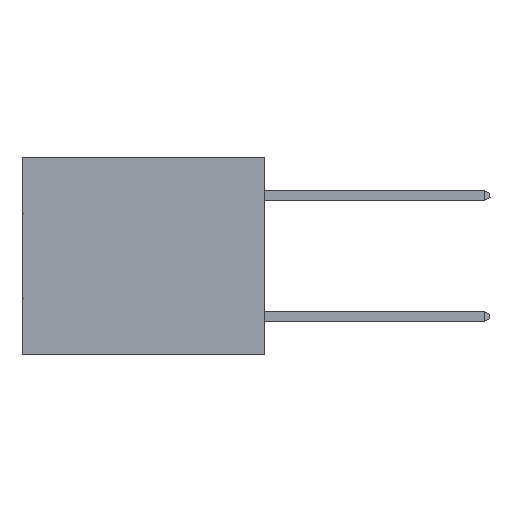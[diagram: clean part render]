
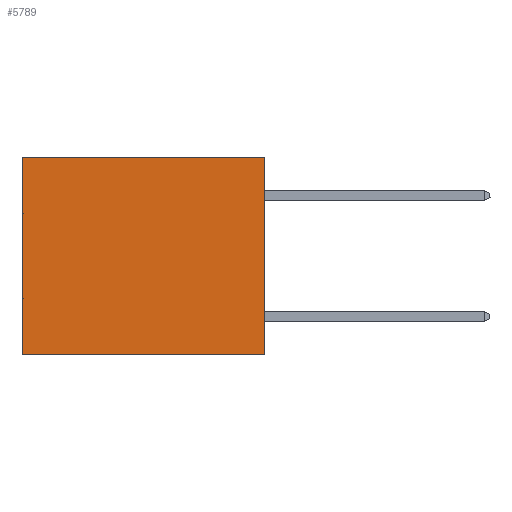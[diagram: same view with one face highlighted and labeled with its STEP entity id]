
A CAD part, left-side view. The second image highlights one B-rep face of the part: STEP entity #5789.
In plain terms, the highlighted planar face has unit normal (-1, 0, 0).
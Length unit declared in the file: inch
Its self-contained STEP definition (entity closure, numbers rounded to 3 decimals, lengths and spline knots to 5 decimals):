
#2473 = EDGE_CURVE ( 'NONE', #23734, #28586, #5473, .T. ) ;
#2545 = VERTEX_POINT ( 'NONE', #25136 ) ;
#4699 = ORIENTED_EDGE ( 'NONE', *, *, #23524, .T. ) ;
#5473 = LINE ( 'NONE', #24772, #13161 ) ;
#5789 = ADVANCED_FACE ( 'NONE', ( #22953 ), #25980, .F. ) ;
#6293 = VECTOR ( 'NONE', #16647, 39.37008 ) ;
#7242 = CARTESIAN_POINT ( 'NONE',  ( 0.3165, 0., 0. ) ) ;
#8237 = EDGE_LOOP ( 'NONE', ( #34367, #9277, #19938, #4699 ) ) ;
#9277 = ORIENTED_EDGE ( 'NONE', *, *, #2473, .F. ) ;
#10460 = LINE ( 'NONE', #29156, #25030 ) ;
#10666 = AXIS2_PLACEMENT_3D ( 'NONE', #26105, #31410, #20607 ) ;
#11845 = CARTESIAN_POINT ( 'NONE',  ( 0.3165, 0.6, -0.49 ) ) ;
#12291 = DIRECTION ( 'NONE',  ( 0., 1., 0. ) ) ;
#12707 = DIRECTION ( 'NONE',  ( 0., 0., -1. ) ) ;
#13161 = VECTOR ( 'NONE', #30084, 39.37008 ) ;
#13885 = CARTESIAN_POINT ( 'NONE',  ( 0.3165, 0.6, -0.49 ) ) ;
#16048 = LINE ( 'NONE', #7242, #27187 ) ;
#16406 = CARTESIAN_POINT ( 'NONE',  ( 0.3165, 0., -0.49 ) ) ;
#16647 = DIRECTION ( 'NONE',  ( 0., 0., -1. ) ) ;
#19938 = ORIENTED_EDGE ( 'NONE', *, *, #22302, .F. ) ;
#20607 = DIRECTION ( 'NONE',  ( 0., 0., -1. ) ) ;
#22302 = EDGE_CURVE ( 'NONE', #2545, #23734, #10460, .T. ) ;
#22953 = FACE_OUTER_BOUND ( 'NONE', #8237, .T. ) ;
#23524 = EDGE_CURVE ( 'NONE', #2545, #27746, #16048, .T. ) ;
#23734 = VERTEX_POINT ( 'NONE', #16406 ) ;
#24772 = CARTESIAN_POINT ( 'NONE',  ( 0.3165, 0., -0.49 ) ) ;
#25030 = VECTOR ( 'NONE', #12707, 39.37008 ) ;
#25136 = CARTESIAN_POINT ( 'NONE',  ( 0.3165, 0., 0. ) ) ;
#25980 = PLANE ( 'NONE',  #10666 ) ;
#26105 = CARTESIAN_POINT ( 'NONE',  ( 0.3165, 0., -0.49 ) ) ;
#27187 = VECTOR ( 'NONE', #12291, 39.37008 ) ;
#27746 = VERTEX_POINT ( 'NONE', #33934 ) ;
#28440 = EDGE_CURVE ( 'NONE', #27746, #28586, #29038, .T. ) ;
#28586 = VERTEX_POINT ( 'NONE', #11845 ) ;
#29038 = LINE ( 'NONE', #13885, #6293 ) ;
#29156 = CARTESIAN_POINT ( 'NONE',  ( 0.3165, 0., -0.49 ) ) ;
#30084 = DIRECTION ( 'NONE',  ( 0., 1., 0. ) ) ;
#31410 = DIRECTION ( 'NONE',  ( 1., 0., 0. ) ) ;
#33934 = CARTESIAN_POINT ( 'NONE',  ( 0.3165, 0.6, 0. ) ) ;
#34367 = ORIENTED_EDGE ( 'NONE', *, *, #28440, .T. ) ;
